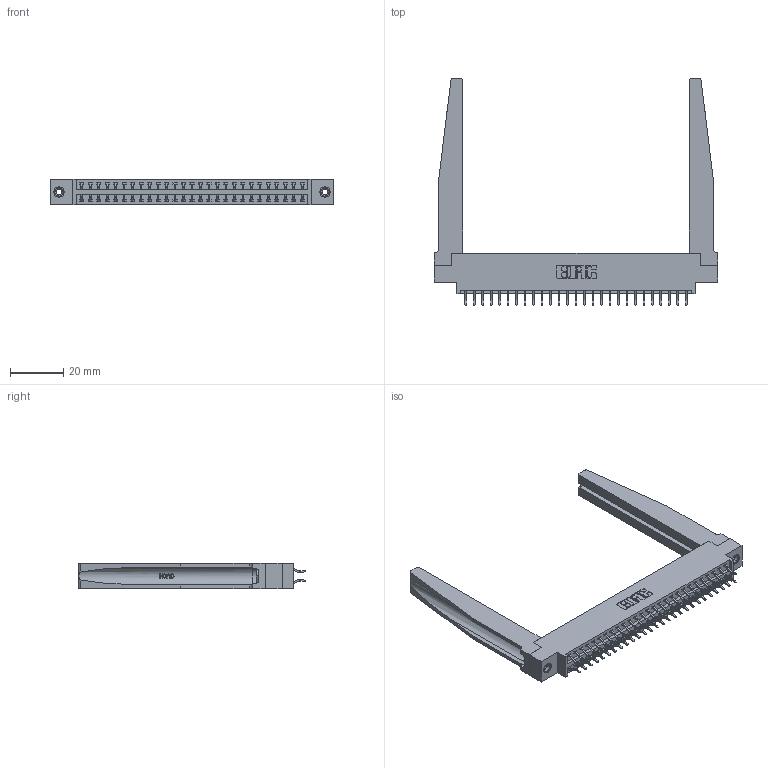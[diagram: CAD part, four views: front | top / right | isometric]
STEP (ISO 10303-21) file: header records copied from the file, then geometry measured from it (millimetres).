
FILE_DESCRIPTION (( 'STEP AP203' ), '1' );
FILE_NAME ('346-054-556-878.STEP', '2022-05-21T04:09:01', ( '' ), ( '' ), 'SwSTEP 2.0', 'SolidWorks 2020', '' );
FILE_SCHEMA (( 'CONFIG_CONTROL_DESIGN' ));
Length unit declared in the file: inch
Products named in the file (5): 345-292-001_556 Tail; 345-250-001_345-250-001-102; 346-220-078_345-220-078; 346 Part_0.170 Offset - 0.156 Dia-TH; 346-054-556-878
Assembly tree (59 placements, depth 2):
  346-054-556-878
    346 Part_0.170 Offset - 0.156 Dia-TH
    345-292-001_556 Tail  x54
    346-220-078_345-220-078  x2
    345-250-001_345-250-001-102  x2
Bounding box: 106.3 x 84.84 x 9.4 mm (x, y, z)
Volume: 16983 mm3; surface area: 20313.3 mm2
Topology: 59 solids, 59 shells, 3506 faces, 10327 edges, 6802 vertices
Faces by surface type: plane 2342, cylinder 1112, bspline 36, cone 12, torus 4
Entity records: 25156 total; most frequent: CARTESIAN_POINT 5125, ORIENTED_EDGE 3934, DIRECTION 3541, EDGE_CURVE 1967, LINE 1625, VECTOR 1625, VERTEX_POINT 1304, AXIS2_PLACEMENT_3D 958
